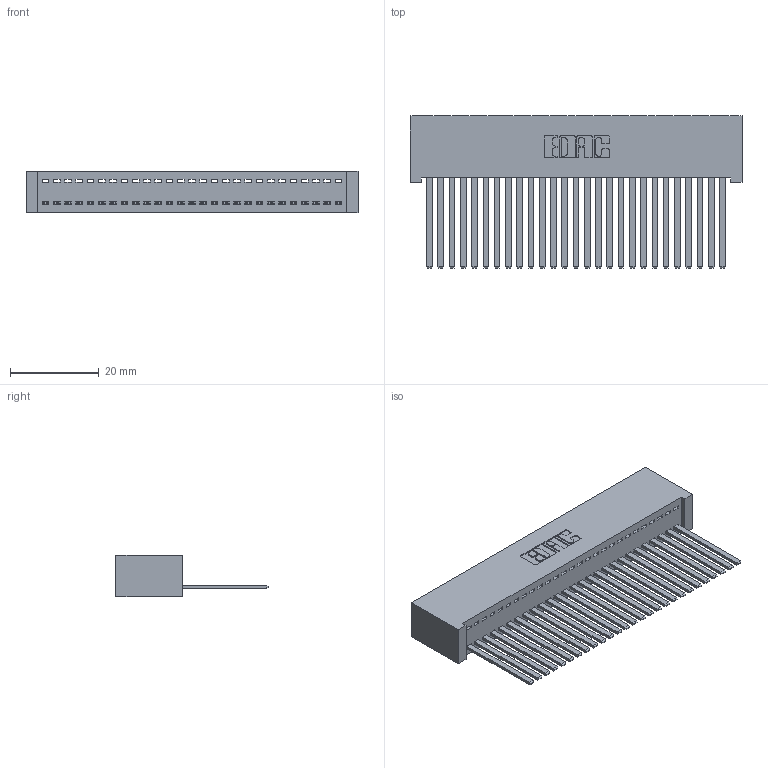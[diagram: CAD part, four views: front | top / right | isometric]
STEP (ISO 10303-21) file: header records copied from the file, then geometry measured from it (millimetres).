
FILE_DESCRIPTION (( 'STEP AP203' ), '1' );
FILE_NAME ('342-027-544-101.STEP', '2019-10-02T02:16:03', ( '' ), ( '' ), 'SwSTEP 2.0', 'SolidWorks 2016', '' );
FILE_SCHEMA (( 'CONFIG_CONTROL_DESIGN' ));
Length unit declared in the file: inch
Products named in the file (3): 345-292-001_345-293-144; 342-027-544-101; 342 Part_Lugless
Assembly tree (28 placements, depth 2):
  342-027-544-101
    342 Part_Lugless
    345-292-001_345-293-144  x27
Bounding box: 74.83 x 34.3 x 9.4 mm (x, y, z)
Volume: 7227.4 mm3; surface area: 11546.3 mm2
Topology: 28 solids, 28 shells, 1506 faces, 4541 edges, 2990 vertices
Faces by surface type: plane 1088, cylinder 418
Entity records: 17853 total; most frequent: CARTESIAN_POINT 3087, ORIENTED_EDGE 3050, DIRECTION 2623, EDGE_CURVE 1525, LINE 1409, VECTOR 1409, VERTEX_POINT 1014, AXIS2_PLACEMENT_3D 607
